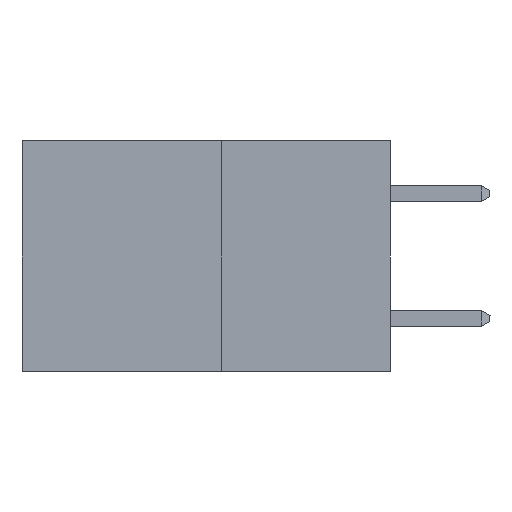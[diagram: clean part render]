
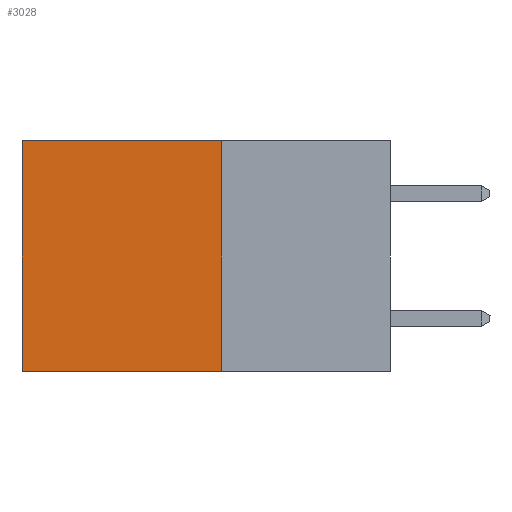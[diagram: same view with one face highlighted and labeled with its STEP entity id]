
A CAD part, left-side view. The second image highlights one B-rep face of the part: STEP entity #3028.
In plain terms, the highlighted planar face has unit normal (-1, 0, 0).
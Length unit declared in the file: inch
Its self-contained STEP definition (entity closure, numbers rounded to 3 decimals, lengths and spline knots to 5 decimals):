
#1896 = CARTESIAN_POINT ( 'NONE',  ( 0.277, 0.59, -0.37 ) ) ;
#2559 = VERTEX_POINT ( 'NONE', #8931 ) ;
#3028 = ADVANCED_FACE ( 'NONE', ( #14996 ), #19343, .F. ) ;
#3062 = LINE ( 'NONE', #3237, #13333 ) ;
#3237 = CARTESIAN_POINT ( 'NONE',  ( 0.277, 0.27, 0. ) ) ;
#3652 = DIRECTION ( 'NONE',  ( 0., 0., -1. ) ) ;
#3928 = VECTOR ( 'NONE', #21893, 39.37008 ) ;
#4167 = ORIENTED_EDGE ( 'NONE', *, *, #7167, .T. ) ;
#5470 = VERTEX_POINT ( 'NONE', #5523 ) ;
#5523 = CARTESIAN_POINT ( 'NONE',  ( 0.277, 0.59, 0. ) ) ;
#6964 = CARTESIAN_POINT ( 'NONE',  ( 0.277, 0.27, -0.37 ) ) ;
#7159 = VECTOR ( 'NONE', #20358, 39.37008 ) ;
#7167 = EDGE_CURVE ( 'NONE', #5470, #14059, #21365, .T. ) ;
#7258 = DIRECTION ( 'NONE',  ( 1., 0., 0. ) ) ;
#7470 = EDGE_CURVE ( 'NONE', #2559, #14059, #19246, .T. ) ;
#7782 = CARTESIAN_POINT ( 'NONE',  ( 0.277, 0.27, 0. ) ) ;
#7818 = ORIENTED_EDGE ( 'NONE', *, *, #23790, .T. ) ;
#8395 = CARTESIAN_POINT ( 'NONE',  ( 0.277, 0.59, -0.37 ) ) ;
#8931 = CARTESIAN_POINT ( 'NONE',  ( 0.277, 0.27, -0.37 ) ) ;
#10402 = EDGE_LOOP ( 'NONE', ( #4167, #21875, #12325, #7818 ) ) ;
#11833 = VECTOR ( 'NONE', #13016, 39.37008 ) ;
#12325 = ORIENTED_EDGE ( 'NONE', *, *, #17780, .F. ) ;
#13016 = DIRECTION ( 'NONE',  ( 0., 0., -1. ) ) ;
#13333 = VECTOR ( 'NONE', #16695, 39.37008 ) ;
#14028 = AXIS2_PLACEMENT_3D ( 'NONE', #22883, #7258, #3652 ) ;
#14059 = VERTEX_POINT ( 'NONE', #1896 ) ;
#14996 = FACE_OUTER_BOUND ( 'NONE', #10402, .T. ) ;
#16695 = DIRECTION ( 'NONE',  ( 0., 1., 0. ) ) ;
#16710 = VERTEX_POINT ( 'NONE', #7782 ) ;
#17780 = EDGE_CURVE ( 'NONE', #16710, #2559, #21834, .T. ) ;
#19246 = LINE ( 'NONE', #23168, #3928 ) ;
#19343 = PLANE ( 'NONE',  #14028 ) ;
#20358 = DIRECTION ( 'NONE',  ( 0., 0., -1. ) ) ;
#21365 = LINE ( 'NONE', #8395, #11833 ) ;
#21834 = LINE ( 'NONE', #6964, #7159 ) ;
#21875 = ORIENTED_EDGE ( 'NONE', *, *, #7470, .F. ) ;
#21893 = DIRECTION ( 'NONE',  ( 0., 1., 0. ) ) ;
#22883 = CARTESIAN_POINT ( 'NONE',  ( 0.277, 0.27, -0.37 ) ) ;
#23168 = CARTESIAN_POINT ( 'NONE',  ( 0.277, 0.27, -0.37 ) ) ;
#23790 = EDGE_CURVE ( 'NONE', #16710, #5470, #3062, .T. ) ;
